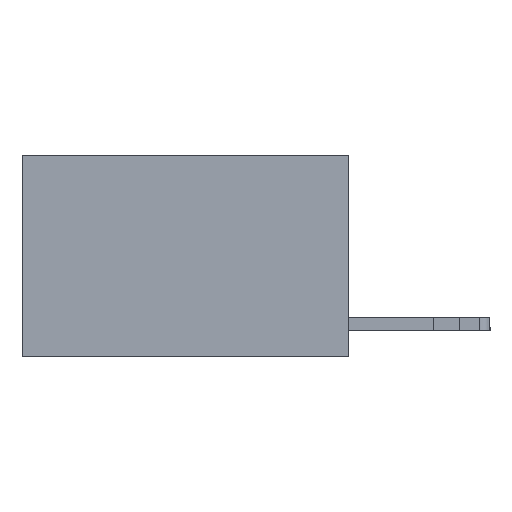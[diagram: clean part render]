
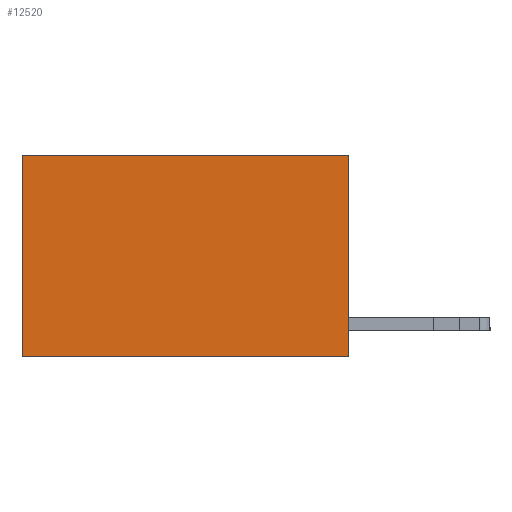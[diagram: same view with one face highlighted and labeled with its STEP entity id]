
A CAD part, left-side view. The second image highlights one B-rep face of the part: STEP entity #12520.
In plain terms, the highlighted planar face has unit normal (-1, 0, 0).
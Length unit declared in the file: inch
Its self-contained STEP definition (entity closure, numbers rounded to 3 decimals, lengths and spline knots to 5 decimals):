
#103 = CARTESIAN_POINT ( 'NONE',  ( 0.2625, 0.6, 0. ) ) ;
#552 = CARTESIAN_POINT ( 'NONE',  ( 0.2625, 0., 0. ) ) ;
#1299 = CARTESIAN_POINT ( 'NONE',  ( 0.2625, 0., 0. ) ) ;
#1546 = PLANE ( 'NONE',  #6086 ) ;
#2194 = ORIENTED_EDGE ( 'NONE', *, *, #11780, .T. ) ;
#2209 = CARTESIAN_POINT ( 'NONE',  ( 0.2625, 0., 0. ) ) ;
#2758 = EDGE_LOOP ( 'NONE', ( #2194, #2849, #6551, #13242 ) ) ;
#2849 = ORIENTED_EDGE ( 'NONE', *, *, #3245, .F. ) ;
#3079 = LINE ( 'NONE', #9291, #9653 ) ;
#3245 = EDGE_CURVE ( 'NONE', #14317, #11697, #3079, .T. ) ;
#3396 = DIRECTION ( 'NONE',  ( 0., 1., 0. ) ) ;
#3919 = CARTESIAN_POINT ( 'NONE',  ( 0.2625, 0., 0. ) ) ;
#5101 = VECTOR ( 'NONE', #9058, 39.37008 ) ;
#5393 = VECTOR ( 'NONE', #3396, 39.37008 ) ;
#6086 = AXIS2_PLACEMENT_3D ( 'NONE', #3919, #8875, #9813 ) ;
#6295 = LINE ( 'NONE', #552, #13616 ) ;
#6551 = ORIENTED_EDGE ( 'NONE', *, *, #13426, .F. ) ;
#6773 = LINE ( 'NONE', #14069, #5101 ) ;
#7747 = VERTEX_POINT ( 'NONE', #103 ) ;
#7831 = CARTESIAN_POINT ( 'NONE',  ( 0.2625, 0., -0.37 ) ) ;
#8875 = DIRECTION ( 'NONE',  ( 1., 0., 0. ) ) ;
#9058 = DIRECTION ( 'NONE',  ( 0., 0., -1. ) ) ;
#9291 = CARTESIAN_POINT ( 'NONE',  ( 0.2625, 0., -0.37 ) ) ;
#9653 = VECTOR ( 'NONE', #15253, 39.37008 ) ;
#9813 = DIRECTION ( 'NONE',  ( 0., 0., -1. ) ) ;
#10165 = CARTESIAN_POINT ( 'NONE',  ( 0.2625, 0.6, -0.37 ) ) ;
#10452 = VERTEX_POINT ( 'NONE', #1299 ) ;
#11151 = FACE_OUTER_BOUND ( 'NONE', #2758, .T. ) ;
#11697 = VERTEX_POINT ( 'NONE', #10165 ) ;
#11780 = EDGE_CURVE ( 'NONE', #7747, #11697, #6773, .T. ) ;
#12520 = ADVANCED_FACE ( 'NONE', ( #11151 ), #1546, .F. ) ;
#12818 = LINE ( 'NONE', #2209, #5393 ) ;
#13242 = ORIENTED_EDGE ( 'NONE', *, *, #15355, .T. ) ;
#13426 = EDGE_CURVE ( 'NONE', #10452, #14317, #6295, .T. ) ;
#13616 = VECTOR ( 'NONE', #14924, 39.37008 ) ;
#14069 = CARTESIAN_POINT ( 'NONE',  ( 0.2625, 0.6, 0. ) ) ;
#14317 = VERTEX_POINT ( 'NONE', #7831 ) ;
#14924 = DIRECTION ( 'NONE',  ( 0., 0., -1. ) ) ;
#15253 = DIRECTION ( 'NONE',  ( 0., 1., 0. ) ) ;
#15355 = EDGE_CURVE ( 'NONE', #10452, #7747, #12818, .T. ) ;
